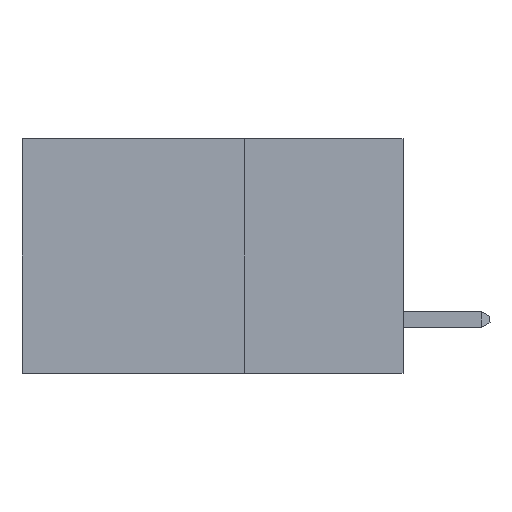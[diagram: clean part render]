
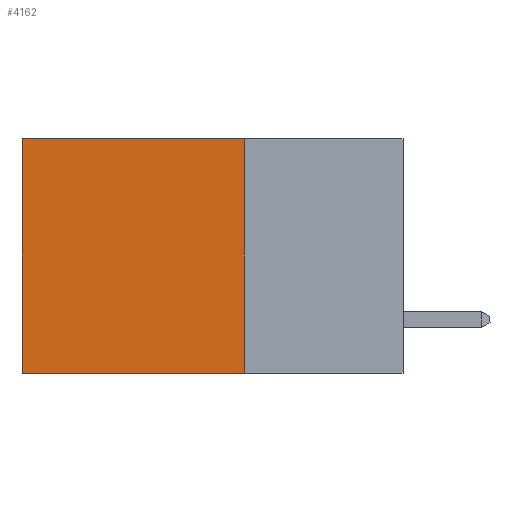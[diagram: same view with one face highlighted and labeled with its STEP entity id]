
A CAD part, left-side view. The second image highlights one B-rep face of the part: STEP entity #4162.
In plain terms, the highlighted planar face has unit normal (-1, 0, 0).
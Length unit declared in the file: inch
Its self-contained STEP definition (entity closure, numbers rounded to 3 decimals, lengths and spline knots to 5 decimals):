
#594 = PLANE ( 'NONE',  #1803 ) ;
#699 = EDGE_CURVE ( 'NONE', #4299, #4850, #11592, .T. ) ;
#1661 = CARTESIAN_POINT ( 'NONE',  ( 0.2875, 0.25, -0.37 ) ) ;
#1683 = EDGE_CURVE ( 'NONE', #4299, #4473, #2333, .T. ) ;
#1763 = DIRECTION ( 'NONE',  ( 1., 0., 0. ) ) ;
#1792 = LINE ( 'NONE', #7060, #4035 ) ;
#1803 = AXIS2_PLACEMENT_3D ( 'NONE', #1829, #1763, #3217 ) ;
#1829 = CARTESIAN_POINT ( 'NONE',  ( 0.2875, 0.25, 0. ) ) ;
#1915 = DIRECTION ( 'NONE',  ( 0., 1., 0. ) ) ;
#2080 = CARTESIAN_POINT ( 'NONE',  ( 0.2875, 0.25, 0. ) ) ;
#2333 = LINE ( 'NONE', #2350, #4852 ) ;
#2350 = CARTESIAN_POINT ( 'NONE',  ( 0.2875, 0.25, 0. ) ) ;
#3018 = CARTESIAN_POINT ( 'NONE',  ( 0.2875, 0.6, 0. ) ) ;
#3217 = DIRECTION ( 'NONE',  ( 0., 0., -1. ) ) ;
#3557 = ORIENTED_EDGE ( 'NONE', *, *, #1683, .T. ) ;
#3558 = VECTOR ( 'NONE', #7240, 39.37008 ) ;
#4035 = VECTOR ( 'NONE', #4305, 39.37008 ) ;
#4162 = ADVANCED_FACE ( 'NONE', ( #5823 ), #594, .F. ) ;
#4299 = VERTEX_POINT ( 'NONE', #2080 ) ;
#4305 = DIRECTION ( 'NONE',  ( 0., 0., -1. ) ) ;
#4435 = EDGE_LOOP ( 'NONE', ( #6385, #6906, #7176, #3557 ) ) ;
#4473 = VERTEX_POINT ( 'NONE', #3018 ) ;
#4850 = VERTEX_POINT ( 'NONE', #6298 ) ;
#4852 = VECTOR ( 'NONE', #1915, 39.37008 ) ;
#4865 = CARTESIAN_POINT ( 'NONE',  ( 0.2875, 0.25, 0. ) ) ;
#5781 = LINE ( 'NONE', #1661, #3558 ) ;
#5823 = FACE_OUTER_BOUND ( 'NONE', #4435, .T. ) ;
#6100 = CARTESIAN_POINT ( 'NONE',  ( 0.2875, 0.6, -0.37 ) ) ;
#6298 = CARTESIAN_POINT ( 'NONE',  ( 0.2875, 0.25, -0.37 ) ) ;
#6385 = ORIENTED_EDGE ( 'NONE', *, *, #8157, .T. ) ;
#6906 = ORIENTED_EDGE ( 'NONE', *, *, #8820, .F. ) ;
#7060 = CARTESIAN_POINT ( 'NONE',  ( 0.2875, 0.6, 0. ) ) ;
#7176 = ORIENTED_EDGE ( 'NONE', *, *, #699, .F. ) ;
#7240 = DIRECTION ( 'NONE',  ( 0., 1., 0. ) ) ;
#8157 = EDGE_CURVE ( 'NONE', #4473, #9250, #1792, .T. ) ;
#8820 = EDGE_CURVE ( 'NONE', #4850, #9250, #5781, .T. ) ;
#9250 = VERTEX_POINT ( 'NONE', #6100 ) ;
#11155 = DIRECTION ( 'NONE',  ( 0., 0., -1. ) ) ;
#11324 = VECTOR ( 'NONE', #11155, 39.37008 ) ;
#11592 = LINE ( 'NONE', #4865, #11324 ) ;
